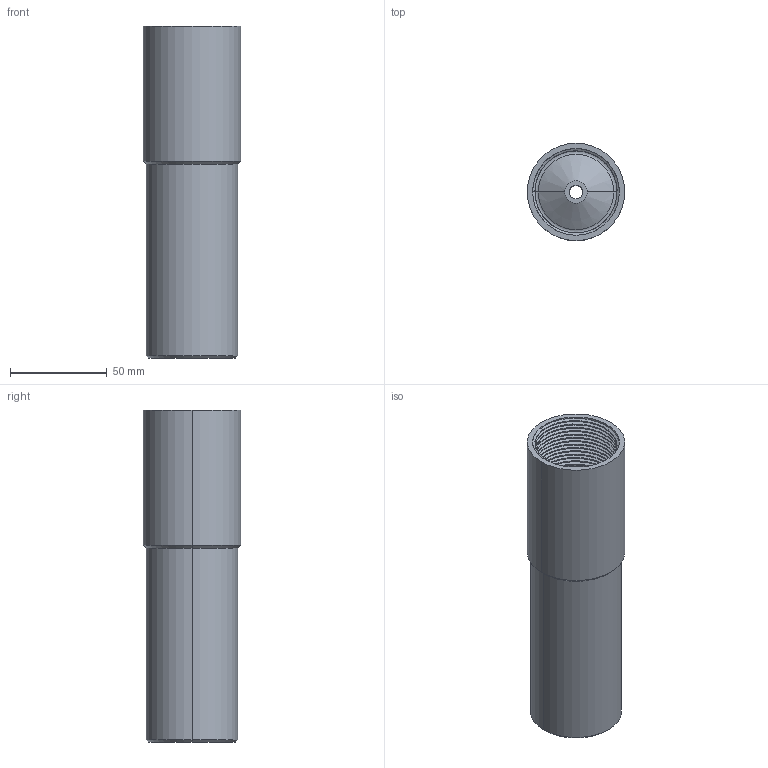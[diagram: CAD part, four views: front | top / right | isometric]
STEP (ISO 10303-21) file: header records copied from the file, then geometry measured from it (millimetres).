
FILE_DESCRIPTION (( 'STEP AP203' ), '1' );
FILE_NAME ('AF-22LRPP-SB-PRT-001-STEP.STEP', '2020-08-29T12:15:52', ( '' ), ( '' ), 'SwSTEP 2.0', 'SolidWorks 2018', '' );
FILE_SCHEMA (( 'CONFIG_CONTROL_DESIGN' ));
Length unit declared in the file: inch
Products named in the file (1): AF-22LRPP-SB-PRT-001-STEP
Bounding box: 50.29 x 50.29 x 171.45 mm (x, y, z)
Volume: 140565.7 mm3; surface area: 102168.9 mm2
Topology: 1 solids, 1 shells, 299 faces, 684 edges, 405 vertices
Faces by surface type: cylinder 110, cone 86, torus 78, plane 22, bspline 3
Entity records: 11156 total; most frequent: CARTESIAN_POINT 4192, DIRECTION 1642, ORIENTED_EDGE 1368, AXIS2_PLACEMENT_3D 719, EDGE_CURVE 684, CIRCLE 422, VERTEX_POINT 405, EDGE_LOOP 319
